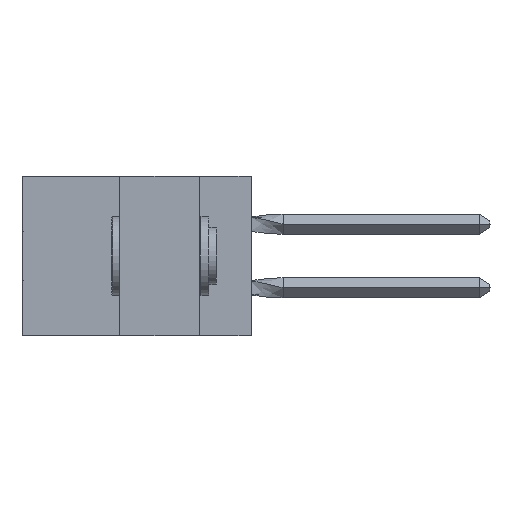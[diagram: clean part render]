
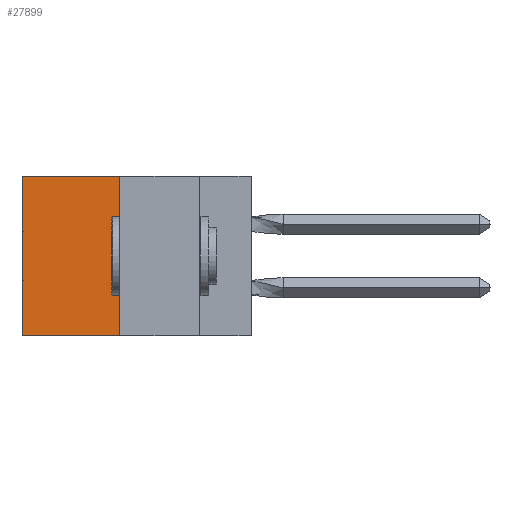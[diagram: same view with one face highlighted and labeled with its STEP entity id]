
A CAD part, left-side view. The second image highlights one B-rep face of the part: STEP entity #27899.
In plain terms, the highlighted planar face has unit normal (-1, 0, 0).
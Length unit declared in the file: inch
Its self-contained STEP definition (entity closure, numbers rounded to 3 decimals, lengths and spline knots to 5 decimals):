
#1379 = LINE ( 'NONE', #41590, #34168 ) ;
#3057 = EDGE_LOOP ( 'NONE', ( #41710, #42259, #14570, #36480 ) ) ;
#6003 = VECTOR ( 'NONE', #11709, 39.37008 ) ;
#6068 = AXIS2_PLACEMENT_3D ( 'NONE', #28565, #25286, #25138 ) ;
#6431 = CARTESIAN_POINT ( 'NONE',  ( 0.305, 0.413, -0.5 ) ) ;
#8818 = VECTOR ( 'NONE', #12400, 39.37008 ) ;
#9025 = EDGE_CURVE ( 'NONE', #27638, #15685, #1379, .T. ) ;
#10484 = LINE ( 'NONE', #32771, #6003 ) ;
#10789 = EDGE_CURVE ( 'NONE', #15685, #26897, #21180, .T. ) ;
#11631 = LINE ( 'NONE', #33633, #8818 ) ;
#11709 = DIRECTION ( 'NONE',  ( 0., 1., 0. ) ) ;
#11736 = CARTESIAN_POINT ( 'NONE',  ( 0.305, 0.72, -0.5 ) ) ;
#12400 = DIRECTION ( 'NONE',  ( 0., 0., -1. ) ) ;
#14570 = ORIENTED_EDGE ( 'NONE', *, *, #42889, .F. ) ;
#15685 = VERTEX_POINT ( 'NONE', #40650 ) ;
#20398 = EDGE_CURVE ( 'NONE', #43230, #26897, #10484, .T. ) ;
#21180 = LINE ( 'NONE', #11736, #44520 ) ;
#24839 = PLANE ( 'NONE',  #6068 ) ;
#25138 = DIRECTION ( 'NONE',  ( 0., 0., -1. ) ) ;
#25286 = DIRECTION ( 'NONE',  ( 1., 0., 0. ) ) ;
#26897 = VERTEX_POINT ( 'NONE', #27530 ) ;
#27530 = CARTESIAN_POINT ( 'NONE',  ( 0.305, 0.72, -0.5 ) ) ;
#27638 = VERTEX_POINT ( 'NONE', #31690 ) ;
#27899 = ADVANCED_FACE ( 'NONE', ( #32844 ), #24839, .F. ) ;
#28565 = CARTESIAN_POINT ( 'NONE',  ( 0.305, 0.413, -0.5 ) ) ;
#31690 = CARTESIAN_POINT ( 'NONE',  ( 0.305, 0.413, 0. ) ) ;
#32771 = CARTESIAN_POINT ( 'NONE',  ( 0.305, 0.413, -0.5 ) ) ;
#32844 = FACE_OUTER_BOUND ( 'NONE', #3057, .T. ) ;
#33633 = CARTESIAN_POINT ( 'NONE',  ( 0.305, 0.413, -0.5 ) ) ;
#33984 = DIRECTION ( 'NONE',  ( 0., 1., 0. ) ) ;
#34168 = VECTOR ( 'NONE', #33984, 39.37008 ) ;
#36480 = ORIENTED_EDGE ( 'NONE', *, *, #9025, .T. ) ;
#40008 = DIRECTION ( 'NONE',  ( 0., 0., -1. ) ) ;
#40650 = CARTESIAN_POINT ( 'NONE',  ( 0.305, 0.72, 0. ) ) ;
#41590 = CARTESIAN_POINT ( 'NONE',  ( 0.305, 0.413, 0. ) ) ;
#41710 = ORIENTED_EDGE ( 'NONE', *, *, #10789, .T. ) ;
#42259 = ORIENTED_EDGE ( 'NONE', *, *, #20398, .F. ) ;
#42889 = EDGE_CURVE ( 'NONE', #27638, #43230, #11631, .T. ) ;
#43230 = VERTEX_POINT ( 'NONE', #6431 ) ;
#44520 = VECTOR ( 'NONE', #40008, 39.37008 ) ;
